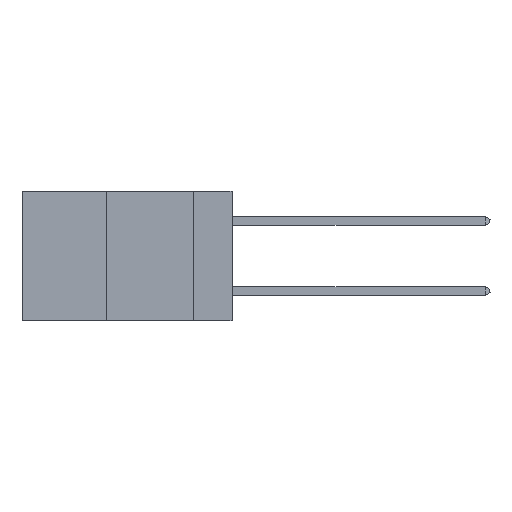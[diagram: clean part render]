
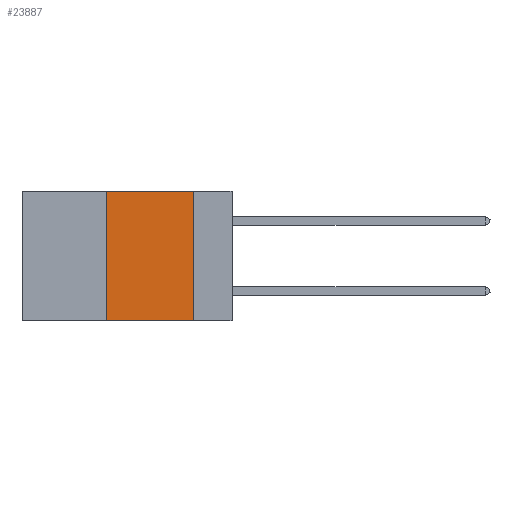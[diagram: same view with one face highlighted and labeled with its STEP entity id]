
A CAD part, left-side view. The second image highlights one B-rep face of the part: STEP entity #23887.
In plain terms, the highlighted planar face has unit normal (-1, 0, 0).
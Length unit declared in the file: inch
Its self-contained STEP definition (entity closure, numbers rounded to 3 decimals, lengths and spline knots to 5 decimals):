
#3635 = PLANE ( 'NONE',  #22439 ) ;
#4513 = VERTEX_POINT ( 'NONE', #42865 ) ;
#7053 = EDGE_CURVE ( 'NONE', #4513, #12050, #35085, .T. ) ;
#8530 = VECTOR ( 'NONE', #25229, 39.37008 ) ;
#8831 = CARTESIAN_POINT ( 'NONE',  ( 0., 0.36, 0. ) ) ;
#10382 = FACE_OUTER_BOUND ( 'NONE', #28460, .T. ) ;
#12050 = VERTEX_POINT ( 'NONE', #36382 ) ;
#12861 = VERTEX_POINT ( 'NONE', #17670 ) ;
#13011 = VECTOR ( 'NONE', #46314, 39.37008 ) ;
#17670 = CARTESIAN_POINT ( 'NONE',  ( 0., 0.11, 0. ) ) ;
#18204 = ORIENTED_EDGE ( 'NONE', *, *, #7053, .T. ) ;
#18691 = ORIENTED_EDGE ( 'NONE', *, *, #43256, .F. ) ;
#19452 = DIRECTION ( 'NONE',  ( 0., 0., -1. ) ) ;
#21892 = LINE ( 'NONE', #37039, #8530 ) ;
#22212 = ORIENTED_EDGE ( 'NONE', *, *, #44950, .F. ) ;
#22439 = AXIS2_PLACEMENT_3D ( 'NONE', #42878, #34531, #19452 ) ;
#23887 = ADVANCED_FACE ( 'NONE', ( #10382 ), #3635, .F. ) ;
#25229 = DIRECTION ( 'NONE',  ( 0., -1., 0. ) ) ;
#26050 = LINE ( 'NONE', #8831, #26646 ) ;
#26646 = VECTOR ( 'NONE', #35812, 39.37008 ) ;
#28460 = EDGE_LOOP ( 'NONE', ( #32801, #18691, #22212, #18204 ) ) ;
#29374 = VECTOR ( 'NONE', #46576, 39.37008 ) ;
#30892 = CARTESIAN_POINT ( 'NONE',  ( 0., 0.11, 0. ) ) ;
#32801 = ORIENTED_EDGE ( 'NONE', *, *, #49890, .F. ) ;
#33134 = VERTEX_POINT ( 'NONE', #33467 ) ;
#33467 = CARTESIAN_POINT ( 'NONE',  ( 0., 0.36, 0. ) ) ;
#34531 = DIRECTION ( 'NONE',  ( 1., 0., 0. ) ) ;
#35085 = LINE ( 'NONE', #38346, #13011 ) ;
#35812 = DIRECTION ( 'NONE',  ( 0., 0., 1. ) ) ;
#36382 = CARTESIAN_POINT ( 'NONE',  ( 0., 0.11, -0.37 ) ) ;
#37039 = CARTESIAN_POINT ( 'NONE',  ( 0., 0.6, 0. ) ) ;
#37916 = LINE ( 'NONE', #30892, #29374 ) ;
#38346 = CARTESIAN_POINT ( 'NONE',  ( 0., 0.6, -0.37 ) ) ;
#42865 = CARTESIAN_POINT ( 'NONE',  ( 0., 0.36, -0.37 ) ) ;
#42878 = CARTESIAN_POINT ( 'NONE',  ( 0., 0.6, 0. ) ) ;
#43256 = EDGE_CURVE ( 'NONE', #33134, #12861, #21892, .T. ) ;
#44950 = EDGE_CURVE ( 'NONE', #4513, #33134, #26050, .T. ) ;
#46314 = DIRECTION ( 'NONE',  ( 0., -1., 0. ) ) ;
#46576 = DIRECTION ( 'NONE',  ( 0., 0., -1. ) ) ;
#49890 = EDGE_CURVE ( 'NONE', #12861, #12050, #37916, .T. ) ;
